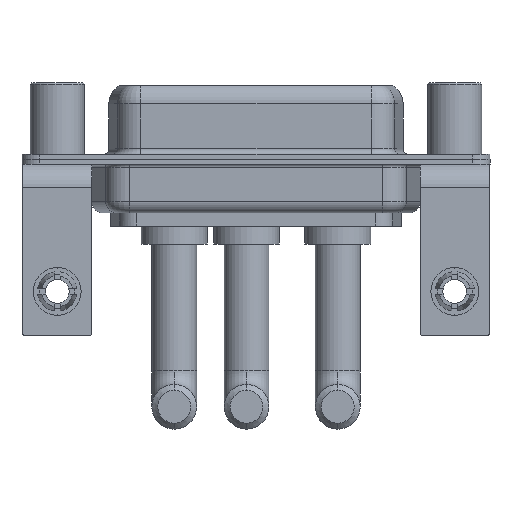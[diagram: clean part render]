
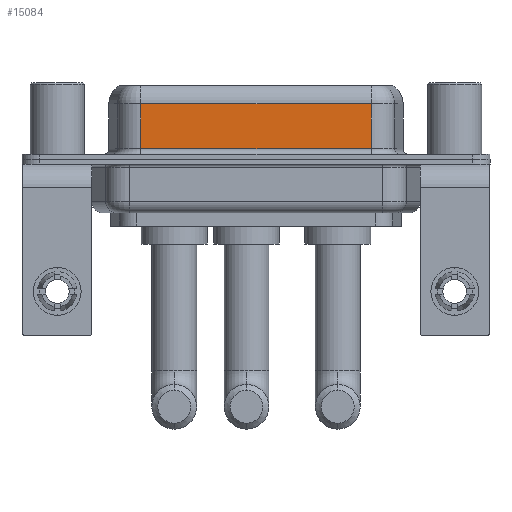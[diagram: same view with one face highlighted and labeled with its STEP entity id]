
A CAD part, front view. The second image highlights one B-rep face of the part: STEP entity #15084.
In plain terms, the highlighted planar face has unit normal (0, -1, 0).
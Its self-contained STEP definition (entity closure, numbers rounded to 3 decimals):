
#839 = LINE ( 'NONE', #3375, #2106 ) ;
#1057 = VERTEX_POINT ( 'NONE', #4418 ) ;
#1274 = EDGE_LOOP ( 'NONE', ( #2213, #15680, #2983, #7231 ) ) ;
#2106 = VECTOR ( 'NONE', #8921, 1000. ) ;
#2213 = ORIENTED_EDGE ( 'NONE', *, *, #11404, .F. ) ;
#2546 = VERTEX_POINT ( 'NONE', #11486 ) ;
#2983 = ORIENTED_EDGE ( 'NONE', *, *, #16937, .T. ) ;
#3235 = AXIS2_PLACEMENT_3D ( 'NONE', #13916, #16794, #15452 ) ;
#3375 = CARTESIAN_POINT ( 'NONE',  ( 7.013, -3.95, 6.4 ) ) ;
#4418 = CARTESIAN_POINT ( 'NONE',  ( 7.013, -3.95, 0.9 ) ) ;
#5032 = CARTESIAN_POINT ( 'NONE',  ( 26.287, -3.95, 0.9 ) ) ;
#5191 = DIRECTION ( 'NONE',  ( 0., 0., -1. ) ) ;
#6433 = EDGE_CURVE ( 'NONE', #1057, #13350, #6883, .T. ) ;
#6454 = CARTESIAN_POINT ( 'NONE',  ( 26.287, -3.95, 6.4 ) ) ;
#6883 = LINE ( 'NONE', #12249, #15512 ) ;
#7094 = PLANE ( 'NONE',  #3235 ) ;
#7231 = ORIENTED_EDGE ( 'NONE', *, *, #6433, .T. ) ;
#7264 = FACE_OUTER_BOUND ( 'NONE', #1274, .T. ) ;
#8921 = DIRECTION ( 'NONE',  ( 0., 0., -1. ) ) ;
#9348 = CARTESIAN_POINT ( 'NONE',  ( 26.287, -3.95, 4.65 ) ) ;
#11246 = VECTOR ( 'NONE', #5191, 1000. ) ;
#11404 = EDGE_CURVE ( 'NONE', #17448, #13350, #17602, .T. ) ;
#11486 = CARTESIAN_POINT ( 'NONE',  ( 7.013, -3.95, 4.65 ) ) ;
#12084 = CARTESIAN_POINT ( 'NONE',  ( 26.287, -3.95, 4.65 ) ) ;
#12249 = CARTESIAN_POINT ( 'NONE',  ( 26.287, -3.95, 0.9 ) ) ;
#12338 = DIRECTION ( 'NONE',  ( 1., 0., 0. ) ) ;
#13350 = VERTEX_POINT ( 'NONE', #5032 ) ;
#13916 = CARTESIAN_POINT ( 'NONE',  ( 26.287, -3.95, 6.4 ) ) ;
#14526 = VECTOR ( 'NONE', #16669, 1000. ) ;
#15084 = ADVANCED_FACE ( 'NONE', ( #7264 ), #7094, .F. ) ;
#15367 = EDGE_CURVE ( 'NONE', #17448, #2546, #17609, .T. ) ;
#15452 = DIRECTION ( 'NONE',  ( 0., 0., 1. ) ) ;
#15512 = VECTOR ( 'NONE', #12338, 1000. ) ;
#15680 = ORIENTED_EDGE ( 'NONE', *, *, #15367, .T. ) ;
#16669 = DIRECTION ( 'NONE',  ( -1., 0., 0. ) ) ;
#16794 = DIRECTION ( 'NONE',  ( 0., 1., 0. ) ) ;
#16937 = EDGE_CURVE ( 'NONE', #2546, #1057, #839, .T. ) ;
#17448 = VERTEX_POINT ( 'NONE', #9348 ) ;
#17602 = LINE ( 'NONE', #6454, #11246 ) ;
#17609 = LINE ( 'NONE', #12084, #14526 ) ;
